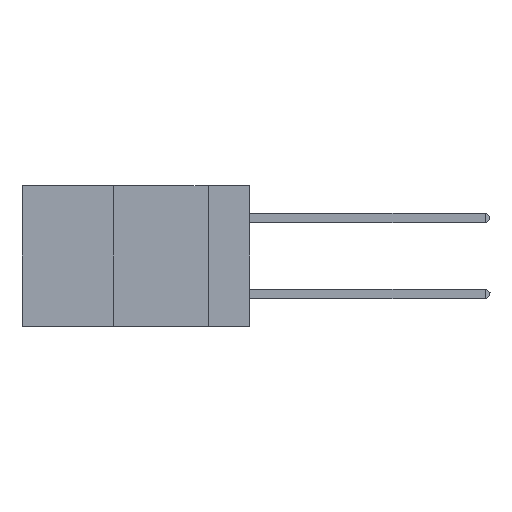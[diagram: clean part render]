
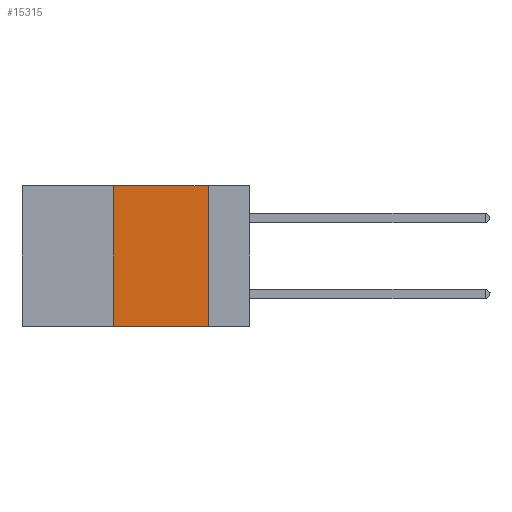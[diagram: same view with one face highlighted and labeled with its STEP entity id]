
A CAD part, left-side view. The second image highlights one B-rep face of the part: STEP entity #15315.
In plain terms, the highlighted planar face has unit normal (-1, 0, 0).
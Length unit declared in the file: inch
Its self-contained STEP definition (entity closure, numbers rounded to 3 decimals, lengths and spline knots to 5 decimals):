
#496 = VERTEX_POINT ( 'NONE', #17681 ) ;
#904 = CARTESIAN_POINT ( 'NONE',  ( 0., 0.11, -0.37 ) ) ;
#997 = EDGE_CURVE ( 'NONE', #496, #16633, #4711, .T. ) ;
#1175 = DIRECTION ( 'NONE',  ( 0., 0., 1. ) ) ;
#1391 = AXIS2_PLACEMENT_3D ( 'NONE', #3221, #6019, #13034 ) ;
#1392 = DIRECTION ( 'NONE',  ( 0., 0., -1. ) ) ;
#1624 = LINE ( 'NONE', #2854, #16078 ) ;
#2550 = FACE_OUTER_BOUND ( 'NONE', #13246, .T. ) ;
#2675 = VECTOR ( 'NONE', #1175, 39.37008 ) ;
#2854 = CARTESIAN_POINT ( 'NONE',  ( 0., 0.11, 0. ) ) ;
#3083 = ORIENTED_EDGE ( 'NONE', *, *, #17442, .T. ) ;
#3221 = CARTESIAN_POINT ( 'NONE',  ( 0., 0.6, 0. ) ) ;
#3890 = ORIENTED_EDGE ( 'NONE', *, *, #13156, .F. ) ;
#4711 = LINE ( 'NONE', #9962, #12521 ) ;
#5686 = DIRECTION ( 'NONE',  ( 0., -1., 0. ) ) ;
#6019 = DIRECTION ( 'NONE',  ( 1., 0., 0. ) ) ;
#6543 = ORIENTED_EDGE ( 'NONE', *, *, #997, .F. ) ;
#6574 = CARTESIAN_POINT ( 'NONE',  ( 0., 0.36, 0. ) ) ;
#7169 = ORIENTED_EDGE ( 'NONE', *, *, #17300, .F. ) ;
#7946 = VERTEX_POINT ( 'NONE', #904 ) ;
#9962 = CARTESIAN_POINT ( 'NONE',  ( 0., 0.6, 0. ) ) ;
#10049 = PLANE ( 'NONE',  #1391 ) ;
#10196 = CARTESIAN_POINT ( 'NONE',  ( 0., 0.11, 0. ) ) ;
#11315 = DIRECTION ( 'NONE',  ( 0., -1., 0. ) ) ;
#12074 = LINE ( 'NONE', #6574, #2675 ) ;
#12521 = VECTOR ( 'NONE', #11315, 39.37008 ) ;
#13034 = DIRECTION ( 'NONE',  ( 0., 0., -1. ) ) ;
#13156 = EDGE_CURVE ( 'NONE', #16633, #7946, #1624, .T. ) ;
#13246 = EDGE_LOOP ( 'NONE', ( #3890, #6543, #7169, #3083 ) ) ;
#13385 = VECTOR ( 'NONE', #5686, 39.37008 ) ;
#14172 = CARTESIAN_POINT ( 'NONE',  ( 0., 0.36, -0.37 ) ) ;
#15315 = ADVANCED_FACE ( 'NONE', ( #2550 ), #10049, .F. ) ;
#16078 = VECTOR ( 'NONE', #1392, 39.37008 ) ;
#16633 = VERTEX_POINT ( 'NONE', #10196 ) ;
#16664 = CARTESIAN_POINT ( 'NONE',  ( 0., 0.6, -0.37 ) ) ;
#17094 = LINE ( 'NONE', #16664, #13385 ) ;
#17300 = EDGE_CURVE ( 'NONE', #17610, #496, #12074, .T. ) ;
#17442 = EDGE_CURVE ( 'NONE', #17610, #7946, #17094, .T. ) ;
#17610 = VERTEX_POINT ( 'NONE', #14172 ) ;
#17681 = CARTESIAN_POINT ( 'NONE',  ( 0., 0.36, 0. ) ) ;
